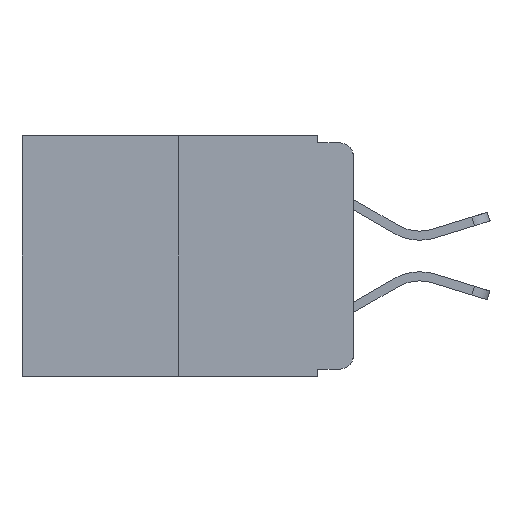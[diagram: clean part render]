
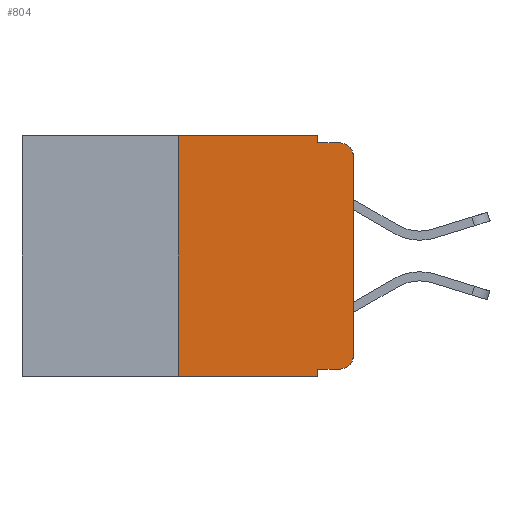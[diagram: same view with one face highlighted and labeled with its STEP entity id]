
A CAD part, left-side view. The second image highlights one B-rep face of the part: STEP entity #804.
In plain terms, the highlighted planar face has unit normal (-1, 0, 0).
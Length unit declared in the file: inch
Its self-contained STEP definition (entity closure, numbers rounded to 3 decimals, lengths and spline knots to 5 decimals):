
#162 = VECTOR ( 'NONE', #14723, 39.37008 ) ;
#759 = EDGE_CURVE ( 'NONE', #17526, #19681, #12213, .T. ) ;
#804 = ADVANCED_FACE ( 'NONE', ( #10518 ), #10374, .F. ) ;
#1167 = EDGE_CURVE ( 'NONE', #15542, #17041, #4352, .T. ) ;
#1232 = LINE ( 'NONE', #8705, #5967 ) ;
#1580 = ORIENTED_EDGE ( 'NONE', *, *, #759, .F. ) ;
#1689 = CARTESIAN_POINT ( 'NONE',  ( 0., 0.051, 0. ) ) ;
#1965 = ORIENTED_EDGE ( 'NONE', *, *, #20104, .T. ) ;
#2047 = CARTESIAN_POINT ( 'NONE',  ( 0., 0.02, -0.01 ) ) ;
#2263 = VECTOR ( 'NONE', #16547, 39.37008 ) ;
#2449 = VECTOR ( 'NONE', #7169, 39.37008 ) ;
#2532 = EDGE_CURVE ( 'NONE', #14600, #17526, #10412, .T. ) ;
#2995 = CARTESIAN_POINT ( 'NONE',  ( 0., 0.473, 0. ) ) ;
#3374 = EDGE_CURVE ( 'NONE', #17238, #11132, #23001, .T. ) ;
#3511 = ORIENTED_EDGE ( 'NONE', *, *, #2532, .F. ) ;
#3712 = CARTESIAN_POINT ( 'NONE',  ( 0., 0.051, -0.01 ) ) ;
#3731 = VECTOR ( 'NONE', #21947, 39.37008 ) ;
#3936 = DIRECTION ( 'NONE',  ( -1., 0., 0. ) ) ;
#4136 = VECTOR ( 'NONE', #12322, 39.37008 ) ;
#4352 = LINE ( 'NONE', #20783, #3731 ) ;
#5631 = ORIENTED_EDGE ( 'NONE', *, *, #19678, .F. ) ;
#5788 = ORIENTED_EDGE ( 'NONE', *, *, #18938, .T. ) ;
#5967 = VECTOR ( 'NONE', #17682, 39.37008 ) ;
#7144 = DIRECTION ( 'NONE',  ( 0., 0., -1. ) ) ;
#7169 = DIRECTION ( 'NONE',  ( 0., -1., 0. ) ) ;
#7501 = ORIENTED_EDGE ( 'NONE', *, *, #1167, .F. ) ;
#7969 = ORIENTED_EDGE ( 'NONE', *, *, #8525, .T. ) ;
#8206 = CARTESIAN_POINT ( 'NONE',  ( 0., 0.051, -0.333 ) ) ;
#8231 = CARTESIAN_POINT ( 'NONE',  ( 0., 0.051, -0.343 ) ) ;
#8525 = EDGE_CURVE ( 'NONE', #10678, #17238, #1232, .T. ) ;
#8705 = CARTESIAN_POINT ( 'NONE',  ( 0., 0., 0. ) ) ;
#9315 = CARTESIAN_POINT ( 'NONE',  ( 0., 0.02, -0.333 ) ) ;
#9360 = VECTOR ( 'NONE', #7144, 39.37008 ) ;
#10374 = PLANE ( 'NONE',  #17513 ) ;
#10412 = LINE ( 'NONE', #13441, #162 ) ;
#10509 = CARTESIAN_POINT ( 'NONE',  ( 0., 0.051, -0.333 ) ) ;
#10518 = FACE_OUTER_BOUND ( 'NONE', #16664, .T. ) ;
#10594 = DIRECTION ( 'NONE',  ( 1., 0., 0. ) ) ;
#10678 = VERTEX_POINT ( 'NONE', #22674 ) ;
#10893 = CARTESIAN_POINT ( 'NONE',  ( 0., 0.051, -0.01 ) ) ;
#11105 = ORIENTED_EDGE ( 'NONE', *, *, #11414, .F. ) ;
#11132 = VERTEX_POINT ( 'NONE', #2047 ) ;
#11286 = DIRECTION ( 'NONE',  ( -1., 0., 0. ) ) ;
#11414 = EDGE_CURVE ( 'NONE', #19681, #21668, #19350, .T. ) ;
#11671 = VECTOR ( 'NONE', #17553, 39.37008 ) ;
#11888 = CARTESIAN_POINT ( 'NONE',  ( 0., 0.473, 0. ) ) ;
#11916 = AXIS2_PLACEMENT_3D ( 'NONE', #15001, #3936, #16754 ) ;
#12213 = LINE ( 'NONE', #2995, #11671 ) ;
#12322 = DIRECTION ( 'NONE',  ( 0., -1., 0. ) ) ;
#12975 = EDGE_CURVE ( 'NONE', #14600, #17041, #16624, .T. ) ;
#13441 = CARTESIAN_POINT ( 'NONE',  ( 0., 0.25, 0. ) ) ;
#14087 = DIRECTION ( 'NONE',  ( 0., 0., -1. ) ) ;
#14600 = VERTEX_POINT ( 'NONE', #16372 ) ;
#14722 = CARTESIAN_POINT ( 'NONE',  ( 0., 0.25, 0. ) ) ;
#14723 = DIRECTION ( 'NONE',  ( 0., 0., 1. ) ) ;
#15001 = CARTESIAN_POINT ( 'NONE',  ( 0., 0.02, -0.03 ) ) ;
#15137 = CIRCLE ( 'NONE', #23195, 0.02 ) ;
#15542 = VERTEX_POINT ( 'NONE', #8206 ) ;
#16372 = CARTESIAN_POINT ( 'NONE',  ( 0., 0.25, -0.343 ) ) ;
#16466 = LINE ( 'NONE', #3712, #2263 ) ;
#16547 = DIRECTION ( 'NONE',  ( 0., -1., 0. ) ) ;
#16624 = LINE ( 'NONE', #19607, #2449 ) ;
#16664 = EDGE_LOOP ( 'NONE', ( #7969, #19067, #5631, #11105, #1580, #3511, #18628, #7501, #1965, #5788 ) ) ;
#16754 = DIRECTION ( 'NONE',  ( 0., 0., -1. ) ) ;
#17041 = VERTEX_POINT ( 'NONE', #8231 ) ;
#17238 = VERTEX_POINT ( 'NONE', #20952 ) ;
#17513 = AXIS2_PLACEMENT_3D ( 'NONE', #11888, #10594, #14087 ) ;
#17526 = VERTEX_POINT ( 'NONE', #14722 ) ;
#17553 = DIRECTION ( 'NONE',  ( 0., -1., 0. ) ) ;
#17682 = DIRECTION ( 'NONE',  ( 0., 0., 1. ) ) ;
#18621 = LINE ( 'NONE', #10509, #4136 ) ;
#18628 = ORIENTED_EDGE ( 'NONE', *, *, #12975, .T. ) ;
#18938 = EDGE_CURVE ( 'NONE', #20380, #10678, #15137, .T. ) ;
#19067 = ORIENTED_EDGE ( 'NONE', *, *, #3374, .T. ) ;
#19350 = LINE ( 'NONE', #19504, #9360 ) ;
#19504 = CARTESIAN_POINT ( 'NONE',  ( 0., 0.051, 0. ) ) ;
#19607 = CARTESIAN_POINT ( 'NONE',  ( 0., 0.473, -0.343 ) ) ;
#19678 = EDGE_CURVE ( 'NONE', #21668, #11132, #16466, .T. ) ;
#19681 = VERTEX_POINT ( 'NONE', #1689 ) ;
#20104 = EDGE_CURVE ( 'NONE', #15542, #20380, #18621, .T. ) ;
#20380 = VERTEX_POINT ( 'NONE', #9315 ) ;
#20783 = CARTESIAN_POINT ( 'NONE',  ( 0., 0.051, 0. ) ) ;
#20952 = CARTESIAN_POINT ( 'NONE',  ( 0., 0., -0.03 ) ) ;
#21668 = VERTEX_POINT ( 'NONE', #10893 ) ;
#21799 = CARTESIAN_POINT ( 'NONE',  ( 0., 0.02, -0.313 ) ) ;
#21947 = DIRECTION ( 'NONE',  ( 0., 0., -1. ) ) ;
#22674 = CARTESIAN_POINT ( 'NONE',  ( 0., 0., -0.313 ) ) ;
#23001 = CIRCLE ( 'NONE', #11916, 0.02 ) ;
#23195 = AXIS2_PLACEMENT_3D ( 'NONE', #21799, #11286, #23503 ) ;
#23503 = DIRECTION ( 'NONE',  ( 0., 0., -1. ) ) ;
